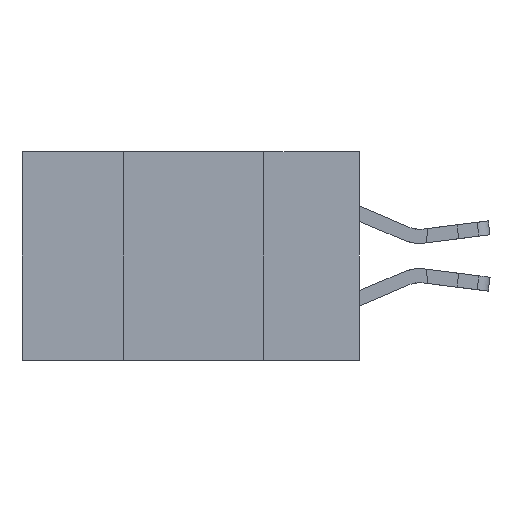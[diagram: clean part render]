
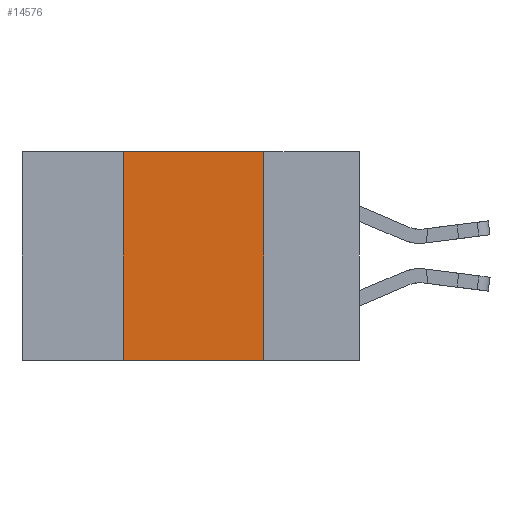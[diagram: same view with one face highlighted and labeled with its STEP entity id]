
A CAD part, left-side view. The second image highlights one B-rep face of the part: STEP entity #14576.
In plain terms, the highlighted planar face has unit normal (-1, 0, 0).
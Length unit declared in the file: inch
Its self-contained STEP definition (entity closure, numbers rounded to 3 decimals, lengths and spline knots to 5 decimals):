
#35 = VECTOR ( 'NONE', #16926, 39.37008 ) ;
#259 = CARTESIAN_POINT ( 'NONE',  ( 0., 0.6, -0.37 ) ) ;
#309 = DIRECTION ( 'NONE',  ( 0., 0., 1. ) ) ;
#352 = VERTEX_POINT ( 'NONE', #3113 ) ;
#600 = VERTEX_POINT ( 'NONE', #18607 ) ;
#3113 = CARTESIAN_POINT ( 'NONE',  ( 0., 0.17, 0. ) ) ;
#4960 = EDGE_CURVE ( 'NONE', #352, #600, #17054, .T. ) ;
#5248 = CARTESIAN_POINT ( 'NONE',  ( 0., 0.42, -0.37 ) ) ;
#5634 = DIRECTION ( 'NONE',  ( 0., 0., -1. ) ) ;
#6064 = DIRECTION ( 'NONE',  ( 1., 0., 0. ) ) ;
#6630 = CARTESIAN_POINT ( 'NONE',  ( 0., 0.42, 0. ) ) ;
#6717 = VERTEX_POINT ( 'NONE', #13958 ) ;
#7262 = EDGE_CURVE ( 'NONE', #6717, #352, #17195, .T. ) ;
#7826 = VECTOR ( 'NONE', #18724, 39.37008 ) ;
#8014 = AXIS2_PLACEMENT_3D ( 'NONE', #13359, #6064, #9081 ) ;
#8550 = LINE ( 'NONE', #259, #7826 ) ;
#8868 = EDGE_CURVE ( 'NONE', #13472, #6717, #13812, .T. ) ;
#9081 = DIRECTION ( 'NONE',  ( 0., 0., -1. ) ) ;
#9266 = CARTESIAN_POINT ( 'NONE',  ( 0., 0.6, 0. ) ) ;
#9440 = FACE_OUTER_BOUND ( 'NONE', #12380, .T. ) ;
#9989 = ORIENTED_EDGE ( 'NONE', *, *, #13150, .T. ) ;
#10246 = PLANE ( 'NONE',  #8014 ) ;
#11829 = ORIENTED_EDGE ( 'NONE', *, *, #8868, .F. ) ;
#12380 = EDGE_LOOP ( 'NONE', ( #14603, #13687, #11829, #9989 ) ) ;
#13150 = EDGE_CURVE ( 'NONE', #13472, #600, #8550, .T. ) ;
#13359 = CARTESIAN_POINT ( 'NONE',  ( 0., 0.6, 0. ) ) ;
#13472 = VERTEX_POINT ( 'NONE', #5248 ) ;
#13687 = ORIENTED_EDGE ( 'NONE', *, *, #7262, .F. ) ;
#13812 = LINE ( 'NONE', #6630, #16526 ) ;
#13958 = CARTESIAN_POINT ( 'NONE',  ( 0., 0.42, 0. ) ) ;
#14576 = ADVANCED_FACE ( 'NONE', ( #9440 ), #10246, .F. ) ;
#14603 = ORIENTED_EDGE ( 'NONE', *, *, #4960, .F. ) ;
#15051 = VECTOR ( 'NONE', #5634, 39.37008 ) ;
#16526 = VECTOR ( 'NONE', #309, 39.37008 ) ;
#16926 = DIRECTION ( 'NONE',  ( 0., -1., 0. ) ) ;
#17054 = LINE ( 'NONE', #17937, #15051 ) ;
#17195 = LINE ( 'NONE', #9266, #35 ) ;
#17937 = CARTESIAN_POINT ( 'NONE',  ( 0., 0.17, 0. ) ) ;
#18607 = CARTESIAN_POINT ( 'NONE',  ( 0., 0.17, -0.37 ) ) ;
#18724 = DIRECTION ( 'NONE',  ( 0., -1., 0. ) ) ;
